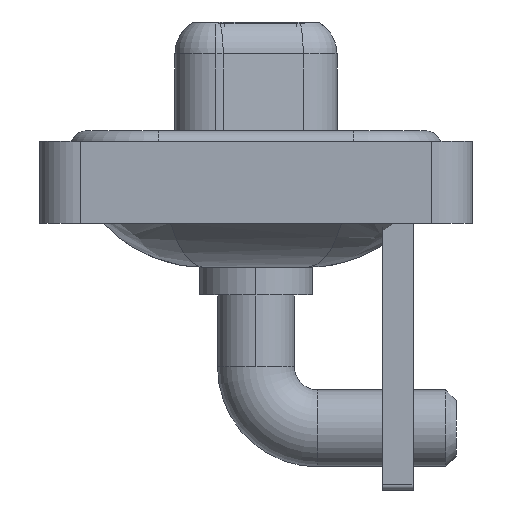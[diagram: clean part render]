
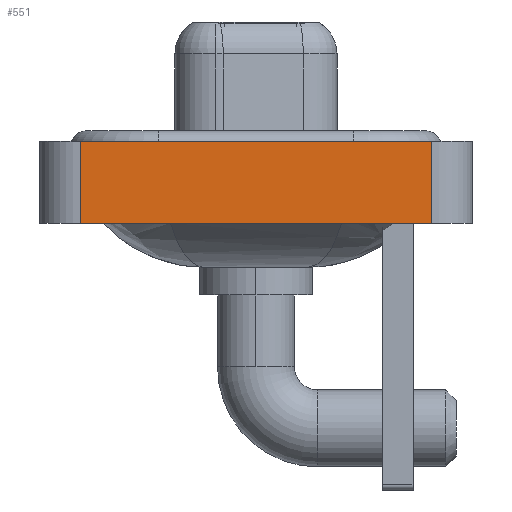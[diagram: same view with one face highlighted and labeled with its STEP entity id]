
A CAD part, left-side view. The second image highlights one B-rep face of the part: STEP entity #551.
In plain terms, the highlighted planar face has unit normal (-1, 0, 0).
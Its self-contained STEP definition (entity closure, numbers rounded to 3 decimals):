
#551 = ADVANCED_FACE ( 'NONE', ( #15049 ), #3032, .T. ) ;
#964 = CARTESIAN_POINT ( 'NONE',  ( -7.35, 8.55, 0.4 ) ) ;
#1095 = VECTOR ( 'NONE', #6709, 1000. ) ;
#1345 = CARTESIAN_POINT ( 'NONE',  ( -7.35, -8.55, -3.6 ) ) ;
#1474 = ORIENTED_EDGE ( 'NONE', *, *, #12723, .T. ) ;
#1631 = EDGE_CURVE ( 'NONE', #13065, #14429, #9404, .T. ) ;
#3032 = PLANE ( 'NONE',  #11055 ) ;
#3250 = EDGE_CURVE ( 'NONE', #3945, #13497, #11823, .T. ) ;
#3687 = CARTESIAN_POINT ( 'NONE',  ( -7.35, 8.55, -3.6 ) ) ;
#3709 = DIRECTION ( 'NONE',  ( 0., 0., 1. ) ) ;
#3875 = CARTESIAN_POINT ( 'NONE',  ( -7.35, 8.55, -3.6 ) ) ;
#3945 = VERTEX_POINT ( 'NONE', #964 ) ;
#4048 = LINE ( 'NONE', #3875, #4384 ) ;
#4384 = VECTOR ( 'NONE', #13264, 1000. ) ;
#5013 = CARTESIAN_POINT ( 'NONE',  ( -7.35, -8.55, 0.4 ) ) ;
#6170 = ORIENTED_EDGE ( 'NONE', *, *, #3250, .F. ) ;
#6709 = DIRECTION ( 'NONE',  ( 0., 0., 1. ) ) ;
#6912 = ORIENTED_EDGE ( 'NONE', *, *, #9478, .F. ) ;
#7053 = ORIENTED_EDGE ( 'NONE', *, *, #1631, .T. ) ;
#7523 = EDGE_LOOP ( 'NONE', ( #1474, #6170, #6912, #7053 ) ) ;
#8397 = CARTESIAN_POINT ( 'NONE',  ( -7.35, -8.55, -3.6 ) ) ;
#9218 = DIRECTION ( 'NONE',  ( 0., -1., 0. ) ) ;
#9404 = LINE ( 'NONE', #14748, #16429 ) ;
#9478 = EDGE_CURVE ( 'NONE', #13065, #3945, #4048, .T. ) ;
#10180 = VECTOR ( 'NONE', #9218, 1000. ) ;
#11055 = AXIS2_PLACEMENT_3D ( 'NONE', #8397, #13718, #3709 ) ;
#11823 = LINE ( 'NONE', #16041, #10180 ) ;
#12723 = EDGE_CURVE ( 'NONE', #14429, #13497, #13367, .T. ) ;
#13065 = VERTEX_POINT ( 'NONE', #3687 ) ;
#13264 = DIRECTION ( 'NONE',  ( 0., 0., 1. ) ) ;
#13367 = LINE ( 'NONE', #1345, #1095 ) ;
#13497 = VERTEX_POINT ( 'NONE', #5013 ) ;
#13718 = DIRECTION ( 'NONE',  ( -1., 0., 0. ) ) ;
#14429 = VERTEX_POINT ( 'NONE', #15900 ) ;
#14748 = CARTESIAN_POINT ( 'NONE',  ( -7.35, -8.55, -3.6 ) ) ;
#15049 = FACE_OUTER_BOUND ( 'NONE', #7523, .T. ) ;
#15900 = CARTESIAN_POINT ( 'NONE',  ( -7.35, -8.55, -3.6 ) ) ;
#16041 = CARTESIAN_POINT ( 'NONE',  ( -7.35, -8.55, 0.4 ) ) ;
#16317 = DIRECTION ( 'NONE',  ( 0., -1., 0. ) ) ;
#16429 = VECTOR ( 'NONE', #16317, 1000. ) ;
